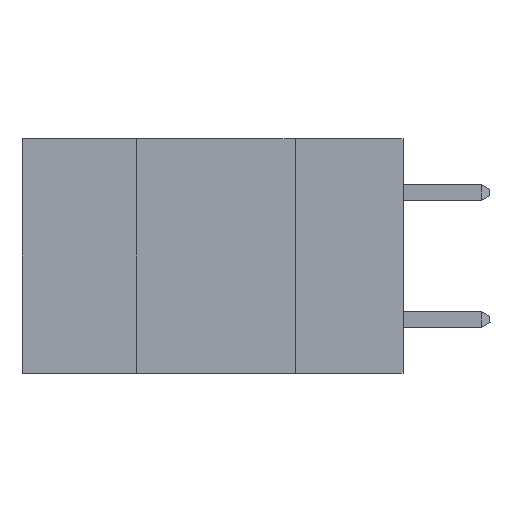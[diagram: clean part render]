
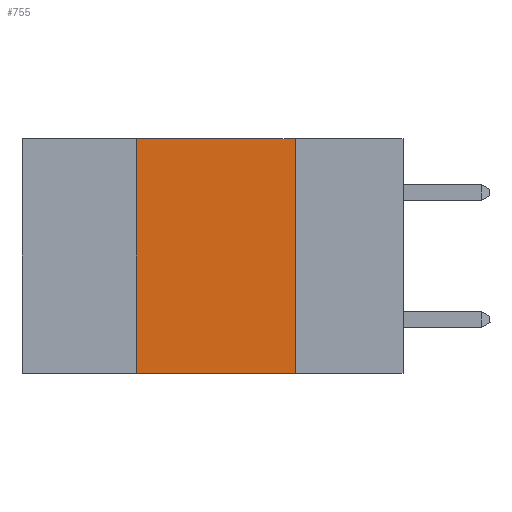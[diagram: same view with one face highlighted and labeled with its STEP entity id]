
A CAD part, left-side view. The second image highlights one B-rep face of the part: STEP entity #755.
In plain terms, the highlighted planar face has unit normal (-1, 0, 0).
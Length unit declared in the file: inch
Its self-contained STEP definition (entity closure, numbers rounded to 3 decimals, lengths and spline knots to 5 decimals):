
#293 = LINE ( 'NONE', #3652, #12277 ) ;
#345 = ORIENTED_EDGE ( 'NONE', *, *, #7593, .F. ) ;
#607 = VERTEX_POINT ( 'NONE', #14582 ) ;
#755 = ADVANCED_FACE ( 'NONE', ( #17467 ), #16506, .F. ) ;
#1086 = LINE ( 'NONE', #5196, #8608 ) ;
#2108 = EDGE_LOOP ( 'NONE', ( #5614, #345, #2653, #14762 ) ) ;
#2553 = EDGE_CURVE ( 'NONE', #607, #11374, #6914, .T. ) ;
#2653 = ORIENTED_EDGE ( 'NONE', *, *, #18942, .F. ) ;
#2700 = DIRECTION ( 'NONE',  ( 1., 0., 0. ) ) ;
#3440 = VERTEX_POINT ( 'NONE', #6514 ) ;
#3652 = CARTESIAN_POINT ( 'NONE',  ( 0., 0.6, 0. ) ) ;
#3851 = VECTOR ( 'NONE', #5552, 39.37008 ) ;
#4866 = CARTESIAN_POINT ( 'NONE',  ( 0., 0.6, 0. ) ) ;
#5196 = CARTESIAN_POINT ( 'NONE',  ( 0., 0.42, 0. ) ) ;
#5552 = DIRECTION ( 'NONE',  ( 0., 0., -1. ) ) ;
#5614 = ORIENTED_EDGE ( 'NONE', *, *, #2553, .F. ) ;
#6514 = CARTESIAN_POINT ( 'NONE',  ( 0., 0.42, 0. ) ) ;
#6914 = LINE ( 'NONE', #10277, #3851 ) ;
#7593 = EDGE_CURVE ( 'NONE', #3440, #607, #293, .T. ) ;
#7845 = CARTESIAN_POINT ( 'NONE',  ( 0., 0.6, -0.37 ) ) ;
#8608 = VECTOR ( 'NONE', #17195, 39.37008 ) ;
#10277 = CARTESIAN_POINT ( 'NONE',  ( 0., 0.17, 0. ) ) ;
#10758 = DIRECTION ( 'NONE',  ( 0., -1., 0. ) ) ;
#11374 = VERTEX_POINT ( 'NONE', #15261 ) ;
#11946 = EDGE_CURVE ( 'NONE', #16665, #11374, #17214, .T. ) ;
#12277 = VECTOR ( 'NONE', #18594, 39.37008 ) ;
#12329 = VECTOR ( 'NONE', #10758, 39.37008 ) ;
#12815 = CARTESIAN_POINT ( 'NONE',  ( 0., 0.42, -0.37 ) ) ;
#14582 = CARTESIAN_POINT ( 'NONE',  ( 0., 0.17, 0. ) ) ;
#14762 = ORIENTED_EDGE ( 'NONE', *, *, #11946, .T. ) ;
#15261 = CARTESIAN_POINT ( 'NONE',  ( 0., 0.17, -0.37 ) ) ;
#16506 = PLANE ( 'NONE',  #18239 ) ;
#16665 = VERTEX_POINT ( 'NONE', #12815 ) ;
#17195 = DIRECTION ( 'NONE',  ( 0., 0., 1. ) ) ;
#17214 = LINE ( 'NONE', #7845, #12329 ) ;
#17467 = FACE_OUTER_BOUND ( 'NONE', #2108, .T. ) ;
#18239 = AXIS2_PLACEMENT_3D ( 'NONE', #4866, #2700, #18845 ) ;
#18594 = DIRECTION ( 'NONE',  ( 0., -1., 0. ) ) ;
#18845 = DIRECTION ( 'NONE',  ( 0., 0., -1. ) ) ;
#18942 = EDGE_CURVE ( 'NONE', #16665, #3440, #1086, .T. ) ;
